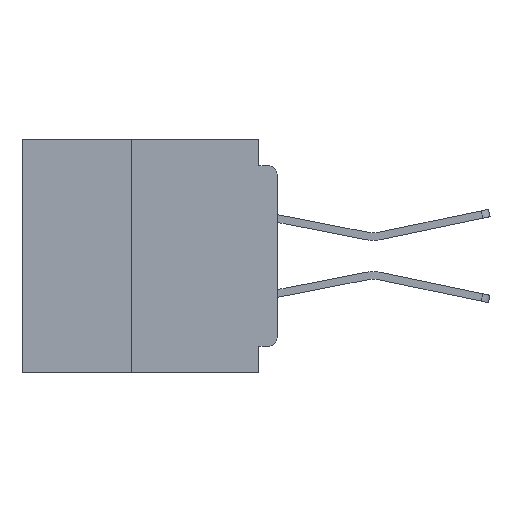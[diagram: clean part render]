
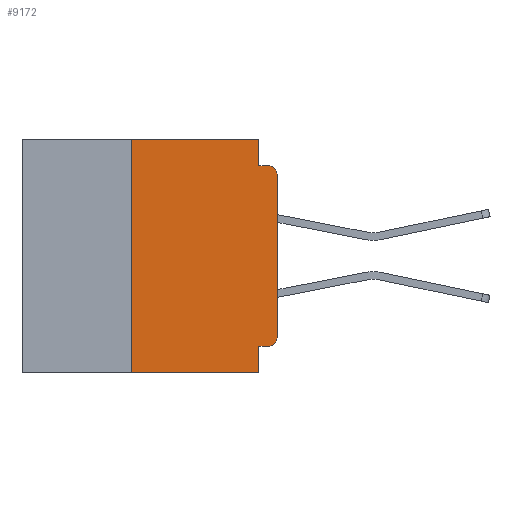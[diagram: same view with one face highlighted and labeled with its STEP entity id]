
A CAD part, left-side view. The second image highlights one B-rep face of the part: STEP entity #9172.
In plain terms, the highlighted planar face has unit normal (-1, 0, 0).
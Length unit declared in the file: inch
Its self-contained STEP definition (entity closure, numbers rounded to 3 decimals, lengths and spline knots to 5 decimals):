
#9 = DIRECTION ( 'NONE',  ( 0., -1., 0. ) ) ;
#58 = VERTEX_POINT ( 'NONE', #19144 ) ;
#973 = VERTEX_POINT ( 'NONE', #33039 ) ;
#1263 = LINE ( 'NONE', #23733, #2420 ) ;
#1355 = DIRECTION ( 'NONE',  ( 0., 0., -1. ) ) ;
#1764 = VERTEX_POINT ( 'NONE', #15971 ) ;
#1850 = DIRECTION ( 'NONE',  ( 0., 0., -1. ) ) ;
#2081 = VECTOR ( 'NONE', #3395, 39.37008 ) ;
#2163 = VECTOR ( 'NONE', #25179, 39.37008 ) ;
#2420 = VECTOR ( 'NONE', #1355, 39.37008 ) ;
#2595 = DIRECTION ( 'NONE',  ( 0., 0., -1. ) ) ;
#3395 = DIRECTION ( 'NONE',  ( 0., 0., -1. ) ) ;
#3536 = DIRECTION ( 'NONE',  ( 0., 0., 1. ) ) ;
#3867 = CARTESIAN_POINT ( 'NONE',  ( 0., 0., 0. ) ) ;
#5052 = EDGE_CURVE ( 'NONE', #38542, #9202, #1263, .T. ) ;
#6925 = EDGE_CURVE ( 'NONE', #37944, #30224, #19324, .T. ) ;
#7941 = CARTESIAN_POINT ( 'NONE',  ( 0., 0., -0.355 ) ) ;
#9172 = ADVANCED_FACE ( 'NONE', ( #10293 ), #43095, .F. ) ;
#9202 = VERTEX_POINT ( 'NONE', #35965 ) ;
#9366 = EDGE_CURVE ( 'NONE', #973, #9202, #39093, .T. ) ;
#9639 = CARTESIAN_POINT ( 'NONE',  ( 0., 0.031, -0.355 ) ) ;
#9890 = EDGE_CURVE ( 'NONE', #27978, #40205, #14940, .T. ) ;
#10293 = FACE_OUTER_BOUND ( 'NONE', #25046, .T. ) ;
#10758 = CARTESIAN_POINT ( 'NONE',  ( 0., 0.031, 0. ) ) ;
#10866 = ORIENTED_EDGE ( 'NONE', *, *, #41254, .F. ) ;
#11416 = LINE ( 'NONE', #10758, #2081 ) ;
#11716 = ORIENTED_EDGE ( 'NONE', *, *, #34133, .F. ) ;
#14449 = CIRCLE ( 'NONE', #42811, 0.015 ) ;
#14940 = CIRCLE ( 'NONE', #30924, 0.015 ) ;
#15473 = AXIS2_PLACEMENT_3D ( 'NONE', #21237, #24973, #2595 ) ;
#15515 = VECTOR ( 'NONE', #3536, 39.37008 ) ;
#15971 = CARTESIAN_POINT ( 'NONE',  ( 0., 0., -0.06 ) ) ;
#17367 = EDGE_CURVE ( 'NONE', #30224, #21969, #11416, .T. ) ;
#17762 = ORIENTED_EDGE ( 'NONE', *, *, #46692, .T. ) ;
#17944 = CARTESIAN_POINT ( 'NONE',  ( 0., 0.015, -0.34 ) ) ;
#18217 = VECTOR ( 'NONE', #22958, 39.37008 ) ;
#19144 = CARTESIAN_POINT ( 'NONE',  ( 0., 0.015, -0.045 ) ) ;
#19324 = LINE ( 'NONE', #41890, #39882 ) ;
#21237 = CARTESIAN_POINT ( 'NONE',  ( 0., 0.437, 0. ) ) ;
#21451 = CARTESIAN_POINT ( 'NONE',  ( 0., 0., -0.045 ) ) ;
#21662 = DIRECTION ( 'NONE',  ( 0., 0., -1. ) ) ;
#21969 = VERTEX_POINT ( 'NONE', #32492 ) ;
#22681 = ORIENTED_EDGE ( 'NONE', *, *, #5052, .F. ) ;
#22958 = DIRECTION ( 'NONE',  ( 0., 1., 0. ) ) ;
#23733 = CARTESIAN_POINT ( 'NONE',  ( 0., 0.031, -0.4 ) ) ;
#24215 = LINE ( 'NONE', #25881, #15515 ) ;
#24234 = DIRECTION ( 'NONE',  ( -1., 0., 0. ) ) ;
#24973 = DIRECTION ( 'NONE',  ( 1., 0., 0. ) ) ;
#25046 = EDGE_LOOP ( 'NONE', ( #40919, #17762, #11716, #40169, #30921, #43022, #37414, #22681, #10866, #35889 ) ) ;
#25179 = DIRECTION ( 'NONE',  ( 0., -1., 0. ) ) ;
#25881 = CARTESIAN_POINT ( 'NONE',  ( 0., 0.25, -0.4 ) ) ;
#26453 = VECTOR ( 'NONE', #29867, 39.37008 ) ;
#27978 = VERTEX_POINT ( 'NONE', #30916 ) ;
#28040 = LINE ( 'NONE', #7941, #18217 ) ;
#29419 = VECTOR ( 'NONE', #9, 39.37008 ) ;
#29867 = DIRECTION ( 'NONE',  ( 0., 0., 1. ) ) ;
#30224 = VERTEX_POINT ( 'NONE', #36606 ) ;
#30916 = CARTESIAN_POINT ( 'NONE',  ( 0., 0.015, -0.355 ) ) ;
#30921 = ORIENTED_EDGE ( 'NONE', *, *, #6925, .F. ) ;
#30924 = AXIS2_PLACEMENT_3D ( 'NONE', #17944, #43511, #21662 ) ;
#30942 = DIRECTION ( 'NONE',  ( 0., -1., 0. ) ) ;
#32019 = CARTESIAN_POINT ( 'NONE',  ( 0., 0.25, 0. ) ) ;
#32492 = CARTESIAN_POINT ( 'NONE',  ( 0., 0.031, -0.045 ) ) ;
#32830 = EDGE_CURVE ( 'NONE', #973, #37944, #24215, .T. ) ;
#32937 = LINE ( 'NONE', #21451, #2163 ) ;
#33039 = CARTESIAN_POINT ( 'NONE',  ( 0., 0.25, -0.4 ) ) ;
#34133 = EDGE_CURVE ( 'NONE', #21969, #58, #32937, .T. ) ;
#34244 = CARTESIAN_POINT ( 'NONE',  ( 0., 0., -0.34 ) ) ;
#35889 = ORIENTED_EDGE ( 'NONE', *, *, #9890, .T. ) ;
#35965 = CARTESIAN_POINT ( 'NONE',  ( 0., 0.031, -0.4 ) ) ;
#36606 = CARTESIAN_POINT ( 'NONE',  ( 0., 0.031, 0. ) ) ;
#37414 = ORIENTED_EDGE ( 'NONE', *, *, #9366, .T. ) ;
#37944 = VERTEX_POINT ( 'NONE', #32019 ) ;
#38542 = VERTEX_POINT ( 'NONE', #9639 ) ;
#39093 = LINE ( 'NONE', #44226, #29419 ) ;
#39882 = VECTOR ( 'NONE', #30942, 39.37008 ) ;
#40169 = ORIENTED_EDGE ( 'NONE', *, *, #17367, .F. ) ;
#40205 = VERTEX_POINT ( 'NONE', #34244 ) ;
#40919 = ORIENTED_EDGE ( 'NONE', *, *, #46406, .T. ) ;
#41254 = EDGE_CURVE ( 'NONE', #27978, #38542, #28040, .T. ) ;
#41890 = CARTESIAN_POINT ( 'NONE',  ( 0., 0.437, 0. ) ) ;
#42811 = AXIS2_PLACEMENT_3D ( 'NONE', #46106, #24234, #1850 ) ;
#43022 = ORIENTED_EDGE ( 'NONE', *, *, #32830, .F. ) ;
#43095 = PLANE ( 'NONE',  #15473 ) ;
#43511 = DIRECTION ( 'NONE',  ( -1., 0., 0. ) ) ;
#44226 = CARTESIAN_POINT ( 'NONE',  ( 0., 0.437, -0.4 ) ) ;
#45853 = LINE ( 'NONE', #3867, #26453 ) ;
#46106 = CARTESIAN_POINT ( 'NONE',  ( 0., 0.015, -0.06 ) ) ;
#46406 = EDGE_CURVE ( 'NONE', #40205, #1764, #45853, .T. ) ;
#46692 = EDGE_CURVE ( 'NONE', #1764, #58, #14449, .T. ) ;
